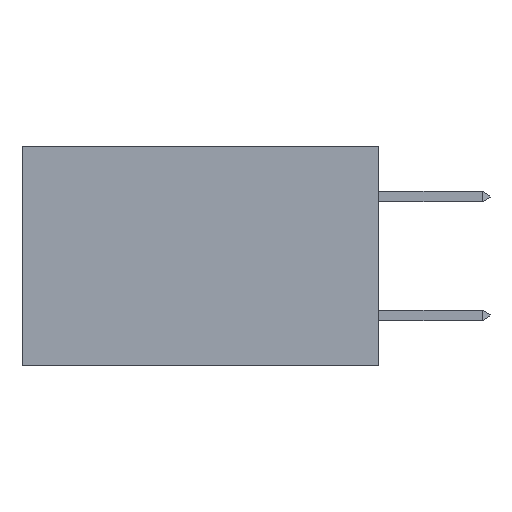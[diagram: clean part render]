
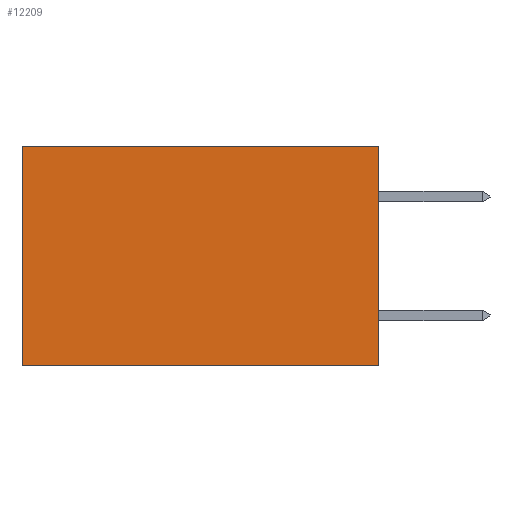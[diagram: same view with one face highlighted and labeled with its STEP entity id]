
A CAD part, left-side view. The second image highlights one B-rep face of the part: STEP entity #12209.
In plain terms, the highlighted planar face has unit normal (-1, 0, 0).
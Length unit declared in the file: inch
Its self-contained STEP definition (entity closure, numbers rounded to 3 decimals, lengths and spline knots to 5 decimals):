
#1616 = VECTOR ( 'NONE', #14375, 39.37008 ) ;
#1825 = ORIENTED_EDGE ( 'NONE', *, *, #19470, .T. ) ;
#3354 = VECTOR ( 'NONE', #19763, 39.37008 ) ;
#3631 = VERTEX_POINT ( 'NONE', #20677 ) ;
#4318 = VERTEX_POINT ( 'NONE', #9820 ) ;
#6006 = ORIENTED_EDGE ( 'NONE', *, *, #7283, .F. ) ;
#6119 = FACE_OUTER_BOUND ( 'NONE', #10704, .T. ) ;
#6211 = DIRECTION ( 'NONE',  ( 1., 0., 0. ) ) ;
#6351 = EDGE_CURVE ( 'NONE', #3631, #4318, #23964, .T. ) ;
#7283 = EDGE_CURVE ( 'NONE', #20126, #22957, #23896, .T. ) ;
#7406 = LINE ( 'NONE', #21080, #3354 ) ;
#9653 = AXIS2_PLACEMENT_3D ( 'NONE', #15468, #6211, #13626 ) ;
#9820 = CARTESIAN_POINT ( 'NONE',  ( 0.298, 0.6, 0. ) ) ;
#10163 = EDGE_CURVE ( 'NONE', #3631, #20126, #21005, .T. ) ;
#10287 = ORIENTED_EDGE ( 'NONE', *, *, #6351, .T. ) ;
#10704 = EDGE_LOOP ( 'NONE', ( #1825, #6006, #12557, #10287 ) ) ;
#11759 = CARTESIAN_POINT ( 'NONE',  ( 0.298, 0., -0.37 ) ) ;
#11821 = PLANE ( 'NONE',  #9653 ) ;
#12209 = ADVANCED_FACE ( 'NONE', ( #6119 ), #11821, .F. ) ;
#12557 = ORIENTED_EDGE ( 'NONE', *, *, #10163, .F. ) ;
#13626 = DIRECTION ( 'NONE',  ( 0., 0., -1. ) ) ;
#13774 = VECTOR ( 'NONE', #22717, 39.37008 ) ;
#14375 = DIRECTION ( 'NONE',  ( 0., 0., -1. ) ) ;
#14393 = VECTOR ( 'NONE', #22273, 39.37008 ) ;
#15151 = CARTESIAN_POINT ( 'NONE',  ( 0.298, 0., -0.37 ) ) ;
#15468 = CARTESIAN_POINT ( 'NONE',  ( 0.298, 0., 0. ) ) ;
#19470 = EDGE_CURVE ( 'NONE', #4318, #22957, #7406, .T. ) ;
#19763 = DIRECTION ( 'NONE',  ( 0., 0., -1. ) ) ;
#20126 = VERTEX_POINT ( 'NONE', #15151 ) ;
#20631 = CARTESIAN_POINT ( 'NONE',  ( 0.298, 0., 0. ) ) ;
#20677 = CARTESIAN_POINT ( 'NONE',  ( 0.298, 0., 0. ) ) ;
#21005 = LINE ( 'NONE', #21732, #1616 ) ;
#21080 = CARTESIAN_POINT ( 'NONE',  ( 0.298, 0.6, 0. ) ) ;
#21732 = CARTESIAN_POINT ( 'NONE',  ( 0.298, 0., 0. ) ) ;
#22227 = CARTESIAN_POINT ( 'NONE',  ( 0.298, 0.6, -0.37 ) ) ;
#22273 = DIRECTION ( 'NONE',  ( 0., 1., 0. ) ) ;
#22717 = DIRECTION ( 'NONE',  ( 0., 1., 0. ) ) ;
#22957 = VERTEX_POINT ( 'NONE', #22227 ) ;
#23896 = LINE ( 'NONE', #11759, #13774 ) ;
#23964 = LINE ( 'NONE', #20631, #14393 ) ;
